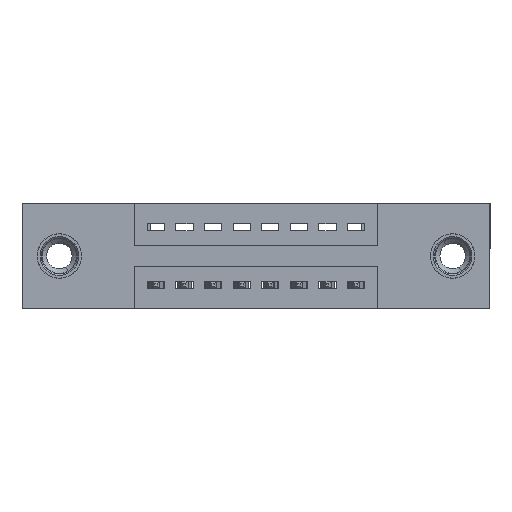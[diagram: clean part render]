
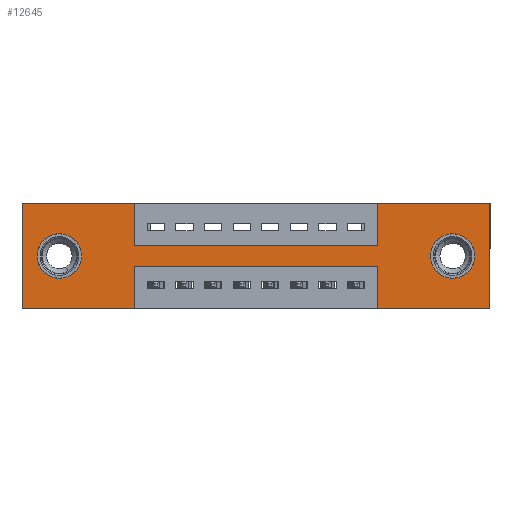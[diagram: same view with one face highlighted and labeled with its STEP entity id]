
A CAD part, front view. The second image highlights one B-rep face of the part: STEP entity #12645.
In plain terms, the highlighted planar face has unit normal (0, -1, 0).
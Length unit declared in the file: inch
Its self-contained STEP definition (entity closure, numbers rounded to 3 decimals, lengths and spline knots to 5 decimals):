
#54 = AXIS2_PLACEMENT_3D ( 'NONE', #4869, #14167, #3522 ) ;
#132 = LINE ( 'NONE', #13843, #4406 ) ;
#178 = ORIENTED_EDGE ( 'NONE', *, *, #7256, .F. ) ;
#195 = EDGE_CURVE ( 'NONE', #681, #10981, #6707, .T. ) ;
#505 = CARTESIAN_POINT ( 'NONE',  ( 0., 0., -0.37 ) ) ;
#585 = VERTEX_POINT ( 'NONE', #13720 ) ;
#672 = DIRECTION ( 'NONE',  ( 0., 0., 1. ) ) ;
#677 = ORIENTED_EDGE ( 'NONE', *, *, #13793, .T. ) ;
#681 = VERTEX_POINT ( 'NONE', #4718 ) ;
#1420 = VECTOR ( 'NONE', #13130, 39.37008 ) ;
#1435 = EDGE_LOOP ( 'NONE', ( #677, #7524 ) ) ;
#1637 = ORIENTED_EDGE ( 'NONE', *, *, #6146, .F. ) ;
#1639 = CARTESIAN_POINT ( 'NONE',  ( 0.3925, 0., -0.22 ) ) ;
#1970 = EDGE_CURVE ( 'NONE', #6975, #14351, #5121, .T. ) ;
#2045 = VECTOR ( 'NONE', #8327, 39.37008 ) ;
#2184 = DIRECTION ( 'NONE',  ( 0., 0., 1. ) ) ;
#2247 = ORIENTED_EDGE ( 'NONE', *, *, #8384, .T. ) ;
#2307 = AXIS2_PLACEMENT_3D ( 'NONE', #8593, #2667, #3951 ) ;
#2397 = VECTOR ( 'NONE', #10614, 39.37008 ) ;
#2531 = ORIENTED_EDGE ( 'NONE', *, *, #1970, .F. ) ;
#2667 = DIRECTION ( 'NONE',  ( 0., 1., 0. ) ) ;
#2675 = EDGE_CURVE ( 'NONE', #4896, #9075, #13445, .T. ) ;
#2760 = EDGE_CURVE ( 'NONE', #12943, #6975, #6366, .T. ) ;
#2837 = EDGE_CURVE ( 'NONE', #11712, #4033, #11193, .T. ) ;
#3052 = CARTESIAN_POINT ( 'NONE',  ( 0.3925, 0., -0.37 ) ) ;
#3107 = VERTEX_POINT ( 'NONE', #14585 ) ;
#3161 = DIRECTION ( 'NONE',  ( 0., 1., 0. ) ) ;
#3198 = CARTESIAN_POINT ( 'NONE',  ( 0.3925, 0., 0. ) ) ;
#3209 = ORIENTED_EDGE ( 'NONE', *, *, #2760, .F. ) ;
#3269 = VECTOR ( 'NONE', #9380, 39.37008 ) ;
#3441 = CARTESIAN_POINT ( 'NONE',  ( 0.3925, 0., 0. ) ) ;
#3522 = DIRECTION ( 'NONE',  ( 0., 0., -1. ) ) ;
#3735 = LINE ( 'NONE', #12186, #6669 ) ;
#3738 = CARTESIAN_POINT ( 'NONE',  ( 1.505, 0., -0.107 ) ) ;
#3784 = LINE ( 'NONE', #5304, #13984 ) ;
#3798 = EDGE_CURVE ( 'NONE', #9075, #14626, #10970, .T. ) ;
#3823 = CARTESIAN_POINT ( 'NONE',  ( 0.13, 0., -0.185 ) ) ;
#3920 = DIRECTION ( 'NONE',  ( -1., 0., 0. ) ) ;
#3928 = ORIENTED_EDGE ( 'NONE', *, *, #8677, .F. ) ;
#3951 = DIRECTION ( 'NONE',  ( 0., 0., -1. ) ) ;
#3980 = EDGE_CURVE ( 'NONE', #585, #4591, #3784, .T. ) ;
#4033 = VERTEX_POINT ( 'NONE', #6257 ) ;
#4155 = ORIENTED_EDGE ( 'NONE', *, *, #3980, .F. ) ;
#4188 = EDGE_LOOP ( 'NONE', ( #2247, #12168 ) ) ;
#4341 = EDGE_LOOP ( 'NONE', ( #15241, #15398, #3928, #15213, #4155, #1637, #6360, #2531, #3209, #178, #11632, #9937 ) ) ;
#4356 = CARTESIAN_POINT ( 'NONE',  ( 1.2425, 0., 0. ) ) ;
#4406 = VECTOR ( 'NONE', #8945, 39.37008 ) ;
#4455 = CARTESIAN_POINT ( 'NONE',  ( 0., 0., -0.37 ) ) ;
#4591 = VERTEX_POINT ( 'NONE', #7777 ) ;
#4718 = CARTESIAN_POINT ( 'NONE',  ( 0.13, 0., -0.263 ) ) ;
#4835 = CARTESIAN_POINT ( 'NONE',  ( 0.3925, 0., -0.15 ) ) ;
#4869 = CARTESIAN_POINT ( 'NONE',  ( 1.505, 0., -0.185 ) ) ;
#4896 = VERTEX_POINT ( 'NONE', #14699 ) ;
#5121 = LINE ( 'NONE', #4835, #1420 ) ;
#5304 = CARTESIAN_POINT ( 'NONE',  ( 1.635, 0., 0. ) ) ;
#5727 = VERTEX_POINT ( 'NONE', #14937 ) ;
#5988 = PLANE ( 'NONE',  #6772 ) ;
#6146 = EDGE_CURVE ( 'NONE', #5727, #585, #14663, .T. ) ;
#6218 = VERTEX_POINT ( 'NONE', #3738 ) ;
#6257 = CARTESIAN_POINT ( 'NONE',  ( 0.3925, 0., -0.22 ) ) ;
#6293 = VECTOR ( 'NONE', #7677, 39.37008 ) ;
#6360 = ORIENTED_EDGE ( 'NONE', *, *, #10214, .F. ) ;
#6366 = LINE ( 'NONE', #3441, #3269 ) ;
#6389 = FACE_BOUND ( 'NONE', #1435, .T. ) ;
#6455 = VECTOR ( 'NONE', #2184, 39.37008 ) ;
#6669 = VECTOR ( 'NONE', #8211, 39.37008 ) ;
#6707 = CIRCLE ( 'NONE', #8241, 0.078 ) ;
#6766 = DIRECTION ( 'NONE',  ( 0., 0., -1. ) ) ;
#6772 = AXIS2_PLACEMENT_3D ( 'NONE', #4455, #13952, #6766 ) ;
#6975 = VERTEX_POINT ( 'NONE', #12653 ) ;
#7022 = VERTEX_POINT ( 'NONE', #9177 ) ;
#7094 = DIRECTION ( 'NONE',  ( -1., 0., 0. ) ) ;
#7211 = DIRECTION ( 'NONE',  ( 0., 0., 1. ) ) ;
#7256 = EDGE_CURVE ( 'NONE', #14626, #12943, #10865, .T. ) ;
#7524 = ORIENTED_EDGE ( 'NONE', *, *, #7710, .T. ) ;
#7677 = DIRECTION ( 'NONE',  ( 0., 0., -1. ) ) ;
#7710 = EDGE_CURVE ( 'NONE', #3107, #6218, #13292, .T. ) ;
#7777 = CARTESIAN_POINT ( 'NONE',  ( 1.635, 0., -0.37 ) ) ;
#7981 = CARTESIAN_POINT ( 'NONE',  ( 0.13, 0., -0.107 ) ) ;
#8019 = VECTOR ( 'NONE', #7211, 39.37008 ) ;
#8211 = DIRECTION ( 'NONE',  ( 0., 0., 1. ) ) ;
#8241 = AXIS2_PLACEMENT_3D ( 'NONE', #14946, #3161, #672 ) ;
#8327 = DIRECTION ( 'NONE',  ( 1., 0., 0. ) ) ;
#8384 = EDGE_CURVE ( 'NONE', #10981, #681, #14704, .T. ) ;
#8593 = CARTESIAN_POINT ( 'NONE',  ( 1.505, 0., -0.185 ) ) ;
#8677 = EDGE_CURVE ( 'NONE', #7022, #11712, #3735, .T. ) ;
#8945 = DIRECTION ( 'NONE',  ( -1., 0., 0. ) ) ;
#8982 = VECTOR ( 'NONE', #7094, 39.37008 ) ;
#8996 = EDGE_CURVE ( 'NONE', #4033, #4896, #10731, .T. ) ;
#9075 = VERTEX_POINT ( 'NONE', #9079 ) ;
#9079 = CARTESIAN_POINT ( 'NONE',  ( 0., 0., -0.37 ) ) ;
#9097 = CARTESIAN_POINT ( 'NONE',  ( 1.2425, 0., -0.22 ) ) ;
#9177 = CARTESIAN_POINT ( 'NONE',  ( 1.2425, 0., -0.37 ) ) ;
#9380 = DIRECTION ( 'NONE',  ( 0., 0., -1. ) ) ;
#9522 = CARTESIAN_POINT ( 'NONE',  ( 0., 0., 0. ) ) ;
#9611 = DIRECTION ( 'NONE',  ( 0., 1., 0. ) ) ;
#9937 = ORIENTED_EDGE ( 'NONE', *, *, #2675, .F. ) ;
#10214 = EDGE_CURVE ( 'NONE', #14351, #5727, #13743, .T. ) ;
#10614 = DIRECTION ( 'NONE',  ( 1., 0., 0. ) ) ;
#10731 = LINE ( 'NONE', #3052, #6293 ) ;
#10865 = LINE ( 'NONE', #13403, #2397 ) ;
#10970 = LINE ( 'NONE', #12934, #8019 ) ;
#10981 = VERTEX_POINT ( 'NONE', #7981 ) ;
#11193 = LINE ( 'NONE', #1639, #13264 ) ;
#11296 = CARTESIAN_POINT ( 'NONE',  ( 0., 0., 0. ) ) ;
#11496 = AXIS2_PLACEMENT_3D ( 'NONE', #3823, #9611, #13363 ) ;
#11632 = ORIENTED_EDGE ( 'NONE', *, *, #3798, .F. ) ;
#11712 = VERTEX_POINT ( 'NONE', #9097 ) ;
#11715 = EDGE_CURVE ( 'NONE', #4591, #7022, #132, .T. ) ;
#12117 = CIRCLE ( 'NONE', #54, 0.078 ) ;
#12168 = ORIENTED_EDGE ( 'NONE', *, *, #195, .T. ) ;
#12186 = CARTESIAN_POINT ( 'NONE',  ( 1.2425, 0., -0.37 ) ) ;
#12483 = DIRECTION ( 'NONE',  ( 0., 0., -1. ) ) ;
#12645 = ADVANCED_FACE ( 'NONE', ( #6389, #13653, #14223 ), #5988, .T. ) ;
#12653 = CARTESIAN_POINT ( 'NONE',  ( 0.3925, 0., -0.15 ) ) ;
#12721 = CARTESIAN_POINT ( 'NONE',  ( 1.2425, 0., -0.15 ) ) ;
#12934 = CARTESIAN_POINT ( 'NONE',  ( 0., 0., 0. ) ) ;
#12943 = VERTEX_POINT ( 'NONE', #3198 ) ;
#13130 = DIRECTION ( 'NONE',  ( 1., 0., 0. ) ) ;
#13264 = VECTOR ( 'NONE', #3920, 39.37008 ) ;
#13292 = CIRCLE ( 'NONE', #2307, 0.078 ) ;
#13363 = DIRECTION ( 'NONE',  ( 0., 0., 1. ) ) ;
#13403 = CARTESIAN_POINT ( 'NONE',  ( 0., 0., 0. ) ) ;
#13445 = LINE ( 'NONE', #505, #8982 ) ;
#13653 = FACE_BOUND ( 'NONE', #4188, .T. ) ;
#13720 = CARTESIAN_POINT ( 'NONE',  ( 1.635, 0., 0. ) ) ;
#13743 = LINE ( 'NONE', #4356, #6455 ) ;
#13793 = EDGE_CURVE ( 'NONE', #6218, #3107, #12117, .T. ) ;
#13843 = CARTESIAN_POINT ( 'NONE',  ( 0., 0., -0.37 ) ) ;
#13952 = DIRECTION ( 'NONE',  ( 0., -1., 0. ) ) ;
#13984 = VECTOR ( 'NONE', #12483, 39.37008 ) ;
#14167 = DIRECTION ( 'NONE',  ( 0., 1., 0. ) ) ;
#14223 = FACE_OUTER_BOUND ( 'NONE', #4341, .T. ) ;
#14351 = VERTEX_POINT ( 'NONE', #12721 ) ;
#14585 = CARTESIAN_POINT ( 'NONE',  ( 1.505, 0., -0.263 ) ) ;
#14626 = VERTEX_POINT ( 'NONE', #11296 ) ;
#14663 = LINE ( 'NONE', #9522, #2045 ) ;
#14699 = CARTESIAN_POINT ( 'NONE',  ( 0.3925, 0., -0.37 ) ) ;
#14704 = CIRCLE ( 'NONE', #11496, 0.078 ) ;
#14937 = CARTESIAN_POINT ( 'NONE',  ( 1.2425, 0., 0. ) ) ;
#14946 = CARTESIAN_POINT ( 'NONE',  ( 0.13, 0., -0.185 ) ) ;
#15213 = ORIENTED_EDGE ( 'NONE', *, *, #11715, .F. ) ;
#15241 = ORIENTED_EDGE ( 'NONE', *, *, #8996, .F. ) ;
#15398 = ORIENTED_EDGE ( 'NONE', *, *, #2837, .F. ) ;
